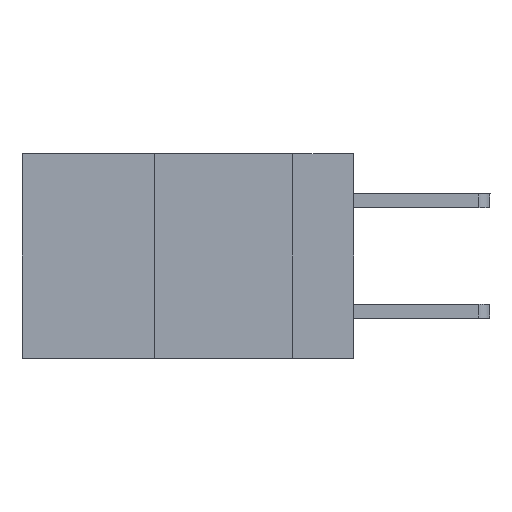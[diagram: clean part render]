
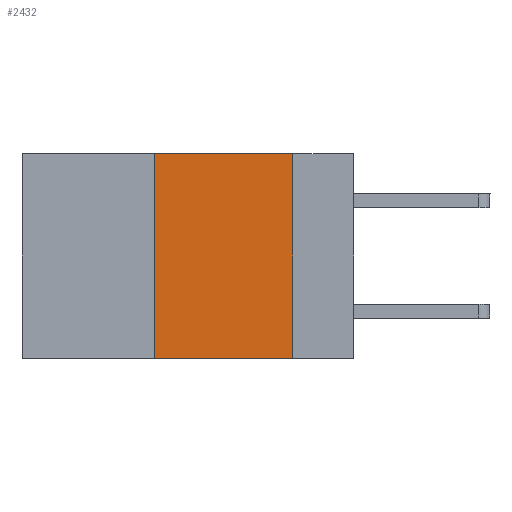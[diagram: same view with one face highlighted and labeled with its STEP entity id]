
A CAD part, left-side view. The second image highlights one B-rep face of the part: STEP entity #2432.
In plain terms, the highlighted planar face has unit normal (-1, 0, 0).
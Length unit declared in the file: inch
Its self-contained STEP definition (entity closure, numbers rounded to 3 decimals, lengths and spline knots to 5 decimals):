
#101 = DIRECTION ( 'NONE',  ( 0., -1., 0. ) ) ;
#366 = VECTOR ( 'NONE', #603, 39.37008 ) ;
#603 = DIRECTION ( 'NONE',  ( 0., 0., -1. ) ) ;
#1062 = VERTEX_POINT ( 'NONE', #10343 ) ;
#1282 = ORIENTED_EDGE ( 'NONE', *, *, #10170, .F. ) ;
#2034 = DIRECTION ( 'NONE',  ( 0., 0., -1. ) ) ;
#2053 = DIRECTION ( 'NONE',  ( 1., 0., 0. ) ) ;
#2119 = CARTESIAN_POINT ( 'NONE',  ( 0., 0.6, 0. ) ) ;
#2134 = PLANE ( 'NONE',  #12041 ) ;
#2432 = ADVANCED_FACE ( 'NONE', ( #8282 ), #2134, .F. ) ;
#2740 = VECTOR ( 'NONE', #14473, 39.37008 ) ;
#4110 = CARTESIAN_POINT ( 'NONE',  ( 0., 0.36, 0. ) ) ;
#4338 = ORIENTED_EDGE ( 'NONE', *, *, #14961, .F. ) ;
#4930 = EDGE_CURVE ( 'NONE', #5242, #9250, #6373, .T. ) ;
#4945 = VERTEX_POINT ( 'NONE', #12251 ) ;
#5153 = CARTESIAN_POINT ( 'NONE',  ( 0., 0.6, -0.37 ) ) ;
#5231 = ORIENTED_EDGE ( 'NONE', *, *, #4930, .F. ) ;
#5242 = VERTEX_POINT ( 'NONE', #10752 ) ;
#5586 = CARTESIAN_POINT ( 'NONE',  ( 0., 0.11, 0. ) ) ;
#6373 = LINE ( 'NONE', #4110, #2740 ) ;
#6546 = CARTESIAN_POINT ( 'NONE',  ( 0., 0.6, 0. ) ) ;
#7004 = LINE ( 'NONE', #5586, #366 ) ;
#7129 = LINE ( 'NONE', #6546, #9494 ) ;
#8282 = FACE_OUTER_BOUND ( 'NONE', #10589, .T. ) ;
#9250 = VERTEX_POINT ( 'NONE', #9795 ) ;
#9297 = EDGE_CURVE ( 'NONE', #5242, #4945, #11976, .T. ) ;
#9494 = VECTOR ( 'NONE', #14592, 39.37008 ) ;
#9795 = CARTESIAN_POINT ( 'NONE',  ( 0., 0.36, 0. ) ) ;
#10170 = EDGE_CURVE ( 'NONE', #9250, #1062, #7129, .T. ) ;
#10343 = CARTESIAN_POINT ( 'NONE',  ( 0., 0.11, 0. ) ) ;
#10553 = ORIENTED_EDGE ( 'NONE', *, *, #9297, .T. ) ;
#10589 = EDGE_LOOP ( 'NONE', ( #4338, #1282, #5231, #10553 ) ) ;
#10752 = CARTESIAN_POINT ( 'NONE',  ( 0., 0.36, -0.37 ) ) ;
#11612 = VECTOR ( 'NONE', #101, 39.37008 ) ;
#11976 = LINE ( 'NONE', #5153, #11612 ) ;
#12041 = AXIS2_PLACEMENT_3D ( 'NONE', #2119, #2053, #2034 ) ;
#12251 = CARTESIAN_POINT ( 'NONE',  ( 0., 0.11, -0.37 ) ) ;
#14473 = DIRECTION ( 'NONE',  ( 0., 0., 1. ) ) ;
#14592 = DIRECTION ( 'NONE',  ( 0., -1., 0. ) ) ;
#14961 = EDGE_CURVE ( 'NONE', #1062, #4945, #7004, .T. ) ;
